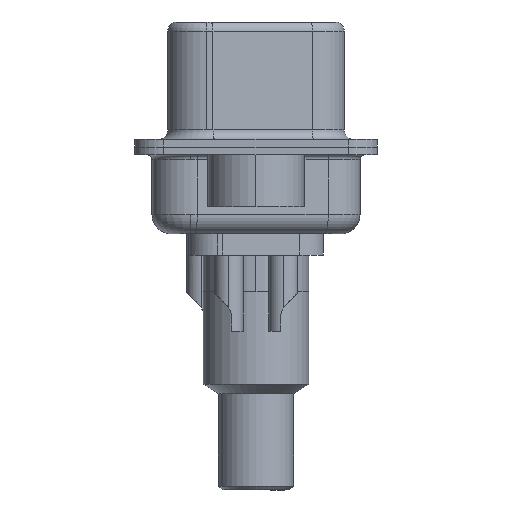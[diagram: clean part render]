
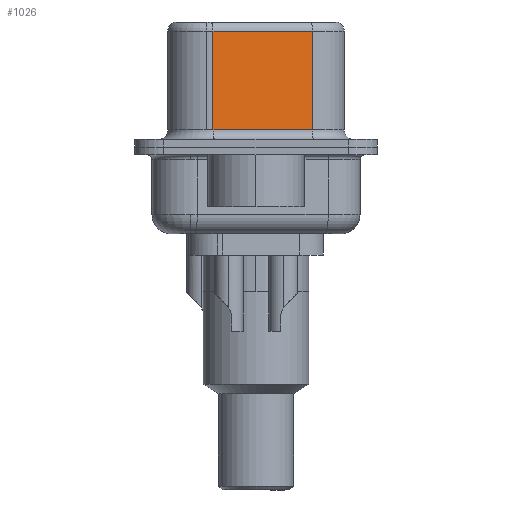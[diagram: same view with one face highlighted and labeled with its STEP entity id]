
A CAD part, left-side view. The second image highlights one B-rep face of the part: STEP entity #1026.
In plain terms, the highlighted planar face has unit normal (-0.985, -0.174, 0).
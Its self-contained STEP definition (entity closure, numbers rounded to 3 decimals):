
#272 = VECTOR ( 'NONE', #3418, 1000. ) ;
#618 = VERTEX_POINT ( 'NONE', #23793 ) ;
#1026 = ADVANCED_FACE ( 'NONE', ( #3356 ), #3246, .F. ) ;
#1729 = EDGE_LOOP ( 'NONE', ( #20383, #14167, #7756, #18047 ) ) ;
#2406 = LINE ( 'NONE', #23722, #14227 ) ;
#3246 = PLANE ( 'NONE',  #11907 ) ;
#3319 = DIRECTION ( 'NONE',  ( -0.174, 0.985, 0. ) ) ;
#3356 = FACE_OUTER_BOUND ( 'NONE', #1729, .T. ) ;
#3418 = DIRECTION ( 'NONE',  ( 0.174, -0.985, 0. ) ) ;
#3756 = CARTESIAN_POINT ( 'NONE',  ( 3.675, 2.233, 0.9 ) ) ;
#4753 = VERTEX_POINT ( 'NONE', #14313 ) ;
#4991 = VERTEX_POINT ( 'NONE', #3756 ) ;
#6430 = CARTESIAN_POINT ( 'NONE',  ( 4.585, -2.927, 6.02 ) ) ;
#6609 = VERTEX_POINT ( 'NONE', #12876 ) ;
#6893 = EDGE_CURVE ( 'NONE', #4753, #618, #11434, .T. ) ;
#7756 = ORIENTED_EDGE ( 'NONE', *, *, #18255, .T. ) ;
#8591 = LINE ( 'NONE', #16505, #272 ) ;
#9195 = DIRECTION ( 'NONE',  ( 0., 0., -1. ) ) ;
#10248 = EDGE_CURVE ( 'NONE', #4753, #6609, #19729, .T. ) ;
#11434 = LINE ( 'NONE', #6430, #23347 ) ;
#11907 = AXIS2_PLACEMENT_3D ( 'NONE', #12320, #18085, #3319 ) ;
#12320 = CARTESIAN_POINT ( 'NONE',  ( 4.585, -2.927, 6.52 ) ) ;
#12876 = CARTESIAN_POINT ( 'NONE',  ( 4.585, -2.927, 0.9 ) ) ;
#14167 = ORIENTED_EDGE ( 'NONE', *, *, #6893, .T. ) ;
#14227 = VECTOR ( 'NONE', #23637, 1000. ) ;
#14313 = CARTESIAN_POINT ( 'NONE',  ( 4.585, -2.927, 6.02 ) ) ;
#16505 = CARTESIAN_POINT ( 'NONE',  ( 4.585, -2.927, 0.9 ) ) ;
#16686 = CARTESIAN_POINT ( 'NONE',  ( 4.585, -2.927, 6.52 ) ) ;
#18047 = ORIENTED_EDGE ( 'NONE', *, *, #22271, .T. ) ;
#18085 = DIRECTION ( 'NONE',  ( 0.985, 0.174, 0. ) ) ;
#18255 = EDGE_CURVE ( 'NONE', #618, #4991, #2406, .T. ) ;
#19534 = DIRECTION ( 'NONE',  ( -0.174, 0.985, 0. ) ) ;
#19729 = LINE ( 'NONE', #16686, #22360 ) ;
#20383 = ORIENTED_EDGE ( 'NONE', *, *, #10248, .F. ) ;
#22271 = EDGE_CURVE ( 'NONE', #4991, #6609, #8591, .T. ) ;
#22360 = VECTOR ( 'NONE', #9195, 1000. ) ;
#23347 = VECTOR ( 'NONE', #19534, 1000. ) ;
#23637 = DIRECTION ( 'NONE',  ( 0., 0., -1. ) ) ;
#23722 = CARTESIAN_POINT ( 'NONE',  ( 3.675, 2.233, 6.52 ) ) ;
#23793 = CARTESIAN_POINT ( 'NONE',  ( 3.675, 2.233, 6.02 ) ) ;
